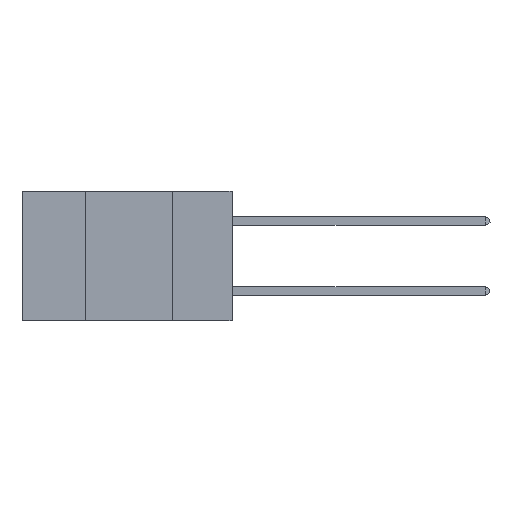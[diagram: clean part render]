
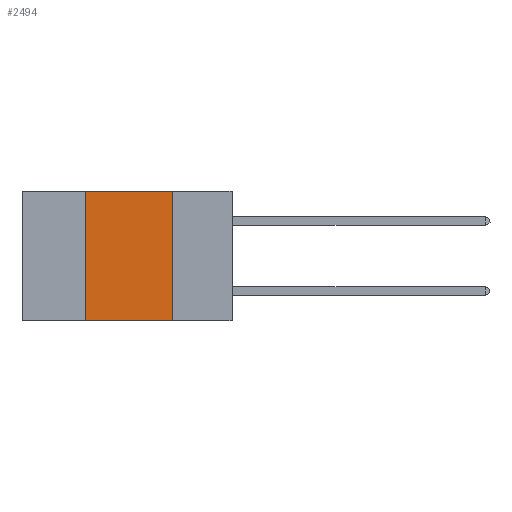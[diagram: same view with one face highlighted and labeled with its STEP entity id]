
A CAD part, left-side view. The second image highlights one B-rep face of the part: STEP entity #2494.
In plain terms, the highlighted planar face has unit normal (-1, 0, 0).
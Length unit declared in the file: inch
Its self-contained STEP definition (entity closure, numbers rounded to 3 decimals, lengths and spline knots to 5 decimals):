
#577 = CARTESIAN_POINT ( 'NONE',  ( 0., 0.17, -0.37 ) ) ;
#1416 = EDGE_LOOP ( 'NONE', ( #12968, #1745, #22902, #2592 ) ) ;
#1481 = CARTESIAN_POINT ( 'NONE',  ( 0., 0.6, 0. ) ) ;
#1745 = ORIENTED_EDGE ( 'NONE', *, *, #20335, .F. ) ;
#2494 = ADVANCED_FACE ( 'NONE', ( #15197 ), #24709, .F. ) ;
#2592 = ORIENTED_EDGE ( 'NONE', *, *, #17442, .T. ) ;
#2707 = EDGE_CURVE ( 'NONE', #19578, #17249, #27159, .T. ) ;
#3089 = CARTESIAN_POINT ( 'NONE',  ( 0., 0.42, 0. ) ) ;
#3333 = DIRECTION ( 'NONE',  ( 0., -1., 0. ) ) ;
#3996 = CARTESIAN_POINT ( 'NONE',  ( 0., 0.42, -0.37 ) ) ;
#4237 = LINE ( 'NONE', #5392, #26265 ) ;
#5271 = AXIS2_PLACEMENT_3D ( 'NONE', #1481, #27015, #22653 ) ;
#5392 = CARTESIAN_POINT ( 'NONE',  ( 0., 0.6, 0. ) ) ;
#8888 = LINE ( 'NONE', #9624, #18517 ) ;
#8943 = CARTESIAN_POINT ( 'NONE',  ( 0., 0.42, 0. ) ) ;
#9624 = CARTESIAN_POINT ( 'NONE',  ( 0., 0.6, -0.37 ) ) ;
#12968 = ORIENTED_EDGE ( 'NONE', *, *, #2707, .F. ) ;
#13792 = LINE ( 'NONE', #8943, #22763 ) ;
#13851 = VECTOR ( 'NONE', #23361, 39.37008 ) ;
#14352 = VERTEX_POINT ( 'NONE', #3996 ) ;
#15197 = FACE_OUTER_BOUND ( 'NONE', #1416, .T. ) ;
#16227 = VERTEX_POINT ( 'NONE', #3089 ) ;
#17249 = VERTEX_POINT ( 'NONE', #577 ) ;
#17442 = EDGE_CURVE ( 'NONE', #14352, #17249, #8888, .T. ) ;
#18517 = VECTOR ( 'NONE', #20347, 39.37008 ) ;
#19578 = VERTEX_POINT ( 'NONE', #23882 ) ;
#19649 = DIRECTION ( 'NONE',  ( 0., 0., 1. ) ) ;
#20335 = EDGE_CURVE ( 'NONE', #16227, #19578, #4237, .T. ) ;
#20347 = DIRECTION ( 'NONE',  ( 0., -1., 0. ) ) ;
#22653 = DIRECTION ( 'NONE',  ( 0., 0., -1. ) ) ;
#22763 = VECTOR ( 'NONE', #19649, 39.37008 ) ;
#22902 = ORIENTED_EDGE ( 'NONE', *, *, #23255, .F. ) ;
#23255 = EDGE_CURVE ( 'NONE', #14352, #16227, #13792, .T. ) ;
#23361 = DIRECTION ( 'NONE',  ( 0., 0., -1. ) ) ;
#23748 = CARTESIAN_POINT ( 'NONE',  ( 0., 0.17, 0. ) ) ;
#23882 = CARTESIAN_POINT ( 'NONE',  ( 0., 0.17, 0. ) ) ;
#24709 = PLANE ( 'NONE',  #5271 ) ;
#26265 = VECTOR ( 'NONE', #3333, 39.37008 ) ;
#27015 = DIRECTION ( 'NONE',  ( 1., 0., 0. ) ) ;
#27159 = LINE ( 'NONE', #23748, #13851 ) ;
